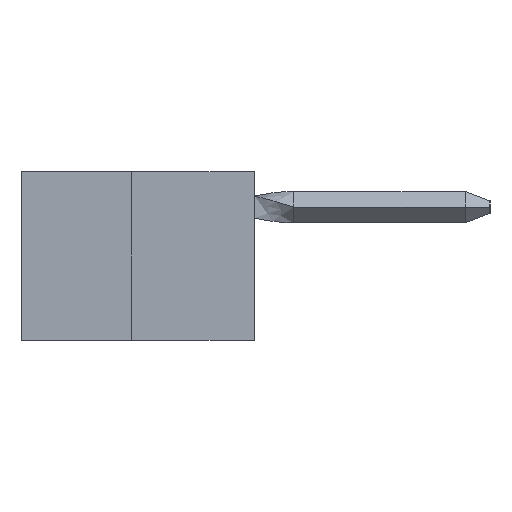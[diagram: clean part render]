
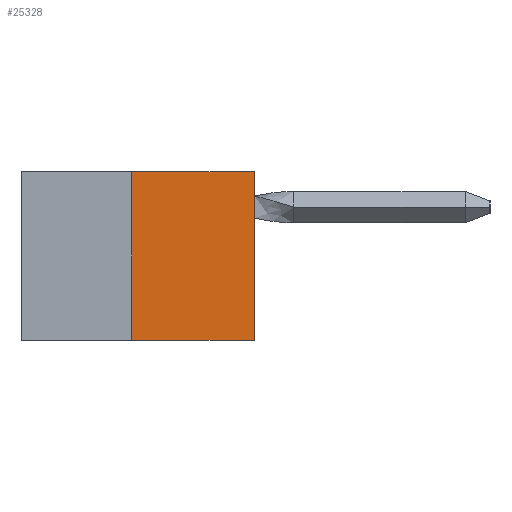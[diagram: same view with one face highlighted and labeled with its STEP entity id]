
A CAD part, left-side view. The second image highlights one B-rep face of the part: STEP entity #25328.
In plain terms, the highlighted planar face has unit normal (-1, 0, 0).
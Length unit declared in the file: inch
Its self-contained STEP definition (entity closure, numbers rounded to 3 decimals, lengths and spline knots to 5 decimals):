
#695 = EDGE_CURVE ( 'NONE', #10184, #19856, #2188, .T. ) ;
#2188 = LINE ( 'NONE', #18521, #29452 ) ;
#2213 = PLANE ( 'NONE',  #26401 ) ;
#2724 = VECTOR ( 'NONE', #11049, 39.37008 ) ;
#3404 = CARTESIAN_POINT ( 'NONE',  ( 0., 0.25, -0.343 ) ) ;
#3833 = CARTESIAN_POINT ( 'NONE',  ( 0., 0.25, 0. ) ) ;
#4423 = FACE_OUTER_BOUND ( 'NONE', #22588, .T. ) ;
#4915 = EDGE_CURVE ( 'NONE', #30335, #19856, #6368, .T. ) ;
#5978 = EDGE_CURVE ( 'NONE', #29677, #30335, #9436, .T. ) ;
#6150 = CARTESIAN_POINT ( 'NONE',  ( 0., 0., 0. ) ) ;
#6368 = LINE ( 'NONE', #26977, #20247 ) ;
#9436 = LINE ( 'NONE', #31263, #2724 ) ;
#10184 = VERTEX_POINT ( 'NONE', #19204 ) ;
#11049 = DIRECTION ( 'NONE',  ( 0., -1., 0. ) ) ;
#11252 = ORIENTED_EDGE ( 'NONE', *, *, #21409, .F. ) ;
#13676 = ORIENTED_EDGE ( 'NONE', *, *, #5978, .T. ) ;
#15450 = ORIENTED_EDGE ( 'NONE', *, *, #695, .F. ) ;
#15678 = ORIENTED_EDGE ( 'NONE', *, *, #4915, .T. ) ;
#18486 = CARTESIAN_POINT ( 'NONE',  ( 0., 0., -0.343 ) ) ;
#18521 = CARTESIAN_POINT ( 'NONE',  ( 0., 0.473, 0. ) ) ;
#19204 = CARTESIAN_POINT ( 'NONE',  ( 0., 0.25, 0. ) ) ;
#19856 = VERTEX_POINT ( 'NONE', #6150 ) ;
#20162 = DIRECTION ( 'NONE',  ( 0., 0., -1. ) ) ;
#20247 = VECTOR ( 'NONE', #31809, 39.37008 ) ;
#21409 = EDGE_CURVE ( 'NONE', #29677, #10184, #27767, .T. ) ;
#22588 = EDGE_LOOP ( 'NONE', ( #15450, #11252, #13676, #15678 ) ) ;
#22606 = CARTESIAN_POINT ( 'NONE',  ( 0., 0.473, 0. ) ) ;
#24085 = DIRECTION ( 'NONE',  ( 0., 0., 1. ) ) ;
#25328 = ADVANCED_FACE ( 'NONE', ( #4423 ), #2213, .F. ) ;
#26401 = AXIS2_PLACEMENT_3D ( 'NONE', #22606, #29846, #20162 ) ;
#26977 = CARTESIAN_POINT ( 'NONE',  ( 0., 0., 0. ) ) ;
#27767 = LINE ( 'NONE', #3833, #29335 ) ;
#29335 = VECTOR ( 'NONE', #24085, 39.37008 ) ;
#29452 = VECTOR ( 'NONE', #31820, 39.37008 ) ;
#29677 = VERTEX_POINT ( 'NONE', #3404 ) ;
#29846 = DIRECTION ( 'NONE',  ( 1., 0., 0. ) ) ;
#30335 = VERTEX_POINT ( 'NONE', #18486 ) ;
#31263 = CARTESIAN_POINT ( 'NONE',  ( 0., 0.473, -0.343 ) ) ;
#31809 = DIRECTION ( 'NONE',  ( 0., 0., 1. ) ) ;
#31820 = DIRECTION ( 'NONE',  ( 0., -1., 0. ) ) ;
